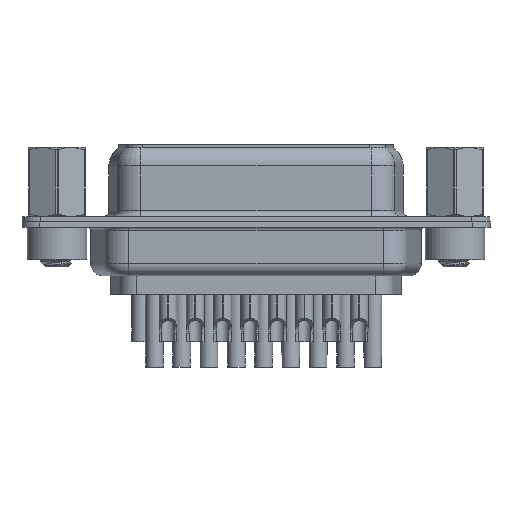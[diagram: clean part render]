
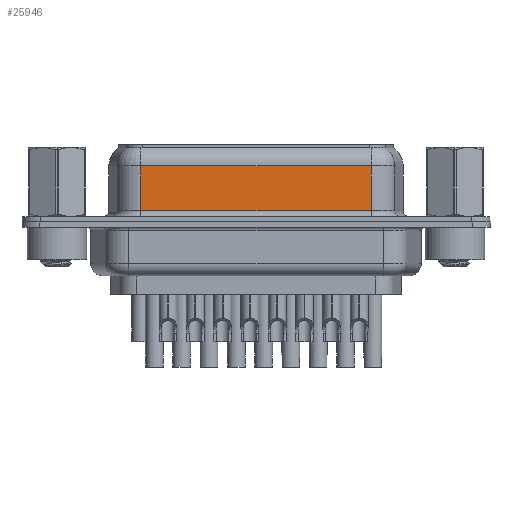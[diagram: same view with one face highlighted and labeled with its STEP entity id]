
A CAD part, front view. The second image highlights one B-rep face of the part: STEP entity #25946.
In plain terms, the highlighted planar face has unit normal (0, -1, 0).
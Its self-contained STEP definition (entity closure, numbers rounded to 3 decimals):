
#786 = DIRECTION ( 'NONE',  ( 1., 0., 0. ) ) ;
#1827 = LINE ( 'NONE', #12266, #3631 ) ;
#2068 = ORIENTED_EDGE ( 'NONE', *, *, #10178, .T. ) ;
#2273 = ORIENTED_EDGE ( 'NONE', *, *, #17259, .T. ) ;
#2409 = LINE ( 'NONE', #9414, #13974 ) ;
#2957 = VECTOR ( 'NONE', #29930, 1000. ) ;
#3631 = VECTOR ( 'NONE', #22359, 1000. ) ;
#6561 = CARTESIAN_POINT ( 'NONE',  ( 7.023, -3.95, 4.7 ) ) ;
#6938 = CARTESIAN_POINT ( 'NONE',  ( 26.297, -3.95, 6.45 ) ) ;
#7450 = DIRECTION ( 'NONE',  ( 0., 1., 0. ) ) ;
#8304 = LINE ( 'NONE', #26640, #20051 ) ;
#8790 = CARTESIAN_POINT ( 'NONE',  ( 7.023, -3.95, 0.95 ) ) ;
#9035 = CARTESIAN_POINT ( 'NONE',  ( 7.023, -3.95, 6.45 ) ) ;
#9187 = ORIENTED_EDGE ( 'NONE', *, *, #13691, .F. ) ;
#9414 = CARTESIAN_POINT ( 'NONE',  ( 26.297, -3.95, 6.45 ) ) ;
#10178 = EDGE_CURVE ( 'NONE', #12975, #11225, #19980, .T. ) ;
#10528 = AXIS2_PLACEMENT_3D ( 'NONE', #6938, #7450, #20472 ) ;
#11225 = VERTEX_POINT ( 'NONE', #8790 ) ;
#11479 = VERTEX_POINT ( 'NONE', #18705 ) ;
#12266 = CARTESIAN_POINT ( 'NONE',  ( 26.297, -3.95, 4.7 ) ) ;
#12975 = VERTEX_POINT ( 'NONE', #6561 ) ;
#13691 = EDGE_CURVE ( 'NONE', #28731, #11479, #2409, .T. ) ;
#13974 = VECTOR ( 'NONE', #30315, 1000. ) ;
#16948 = EDGE_CURVE ( 'NONE', #11225, #11479, #8304, .T. ) ;
#17259 = EDGE_CURVE ( 'NONE', #28731, #12975, #1827, .T. ) ;
#18705 = CARTESIAN_POINT ( 'NONE',  ( 26.297, -3.95, 0.95 ) ) ;
#19980 = LINE ( 'NONE', #9035, #2957 ) ;
#20051 = VECTOR ( 'NONE', #786, 1000. ) ;
#20472 = DIRECTION ( 'NONE',  ( 0., 0., 1. ) ) ;
#22359 = DIRECTION ( 'NONE',  ( -1., 0., 0. ) ) ;
#23025 = PLANE ( 'NONE',  #10528 ) ;
#25946 = ADVANCED_FACE ( 'NONE', ( #28357 ), #23025, .F. ) ;
#26640 = CARTESIAN_POINT ( 'NONE',  ( 26.297, -3.95, 0.95 ) ) ;
#28357 = FACE_OUTER_BOUND ( 'NONE', #29592, .T. ) ;
#28731 = VERTEX_POINT ( 'NONE', #32083 ) ;
#29592 = EDGE_LOOP ( 'NONE', ( #9187, #2273, #2068, #31206 ) ) ;
#29930 = DIRECTION ( 'NONE',  ( 0., 0., -1. ) ) ;
#30315 = DIRECTION ( 'NONE',  ( 0., 0., -1. ) ) ;
#31206 = ORIENTED_EDGE ( 'NONE', *, *, #16948, .T. ) ;
#32083 = CARTESIAN_POINT ( 'NONE',  ( 26.297, -3.95, 4.7 ) ) ;
